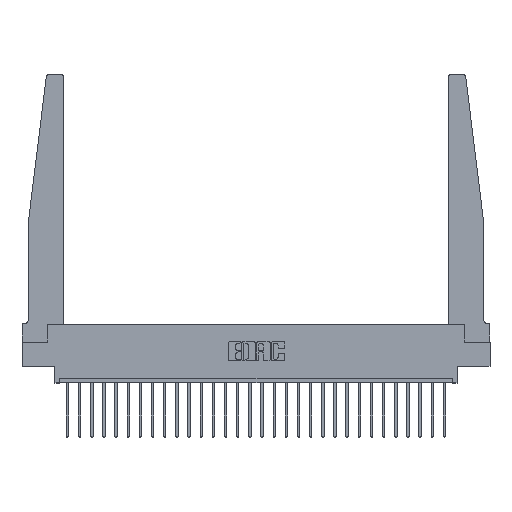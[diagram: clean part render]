
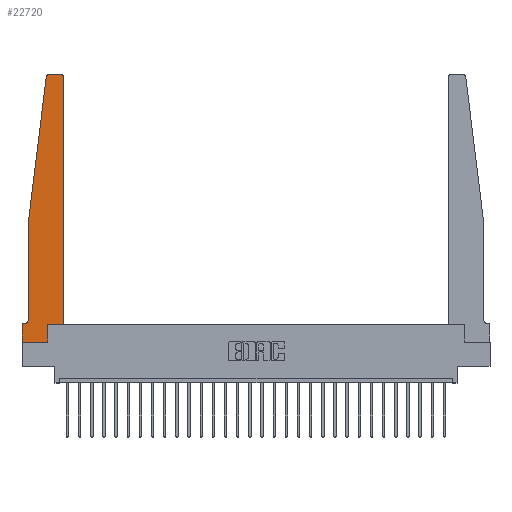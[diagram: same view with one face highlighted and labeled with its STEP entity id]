
A CAD part, top view. The second image highlights one B-rep face of the part: STEP entity #22720.
In plain terms, the highlighted planar face has unit normal (0, 0, 1).
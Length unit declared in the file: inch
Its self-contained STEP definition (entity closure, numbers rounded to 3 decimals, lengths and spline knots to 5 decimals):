
#14 = AXIS2_PLACEMENT_3D ( 'NONE', #17713, #17983, #10589 ) ;
#166 = VERTEX_POINT ( 'NONE', #11202 ) ;
#487 = CARTESIAN_POINT ( 'NONE',  ( 0., 0.1875, 0.37 ) ) ;
#514 = VECTOR ( 'NONE', #20784, 39.37008 ) ;
#967 = VERTEX_POINT ( 'NONE', #8251 ) ;
#980 = ORIENTED_EDGE ( 'NONE', *, *, #1499, .T. ) ;
#1088 = LINE ( 'NONE', #23328, #3349 ) ;
#1499 = EDGE_CURVE ( 'NONE', #7745, #23805, #2889, .T. ) ;
#1550 = CARTESIAN_POINT ( 'NONE',  ( 0.25, 2.75, 0.37 ) ) ;
#1718 = AXIS2_PLACEMENT_3D ( 'NONE', #17797, #5734, #7734 ) ;
#1738 = LINE ( 'NONE', #13025, #6844 ) ;
#2017 = ORIENTED_EDGE ( 'NONE', *, *, #8646, .T. ) ;
#2110 = DIRECTION ( 'NONE',  ( -1., 0., 0. ) ) ;
#2233 = VECTOR ( 'NONE', #14215, 39.37008 ) ;
#2363 = ORIENTED_EDGE ( 'NONE', *, *, #16042, .T. ) ;
#2469 = DIRECTION ( 'NONE',  ( 0., 0., 1. ) ) ;
#2528 = CARTESIAN_POINT ( 'NONE',  ( 0., 0., 0.37 ) ) ;
#2587 = VECTOR ( 'NONE', #2110, 39.37008 ) ;
#2889 = LINE ( 'NONE', #1550, #2587 ) ;
#3087 = ORIENTED_EDGE ( 'NONE', *, *, #20840, .T. ) ;
#3349 = VECTOR ( 'NONE', #17210, 39.37008 ) ;
#4024 = LINE ( 'NONE', #2528, #514 ) ;
#4312 = VECTOR ( 'NONE', #16308, 39.37008 ) ;
#4846 = EDGE_CURVE ( 'NONE', #10331, #13858, #1738, .T. ) ;
#5045 = EDGE_CURVE ( 'NONE', #23805, #17679, #9657, .T. ) ;
#5103 = ORIENTED_EDGE ( 'NONE', *, *, #4846, .T. ) ;
#5146 = DIRECTION ( 'NONE',  ( 0., 1., 0. ) ) ;
#5177 = VECTOR ( 'NONE', #21543, 39.37008 ) ;
#5707 = EDGE_CURVE ( 'NONE', #23766, #21715, #9662, .T. ) ;
#5734 = DIRECTION ( 'NONE',  ( 0., 0., -1. ) ) ;
#5841 = VERTEX_POINT ( 'NONE', #16495 ) ;
#5907 = EDGE_CURVE ( 'NONE', #17679, #967, #1088, .T. ) ;
#6087 = ORIENTED_EDGE ( 'NONE', *, *, #5907, .T. ) ;
#6761 = ORIENTED_EDGE ( 'NONE', *, *, #5707, .T. ) ;
#6844 = VECTOR ( 'NONE', #12948, 39.37008 ) ;
#7000 = EDGE_CURVE ( 'NONE', #967, #19310, #20351, .T. ) ;
#7734 = DIRECTION ( 'NONE',  ( -1., 0., 0. ) ) ;
#7745 = VERTEX_POINT ( 'NONE', #17360 ) ;
#7827 = PLANE ( 'NONE',  #14 ) ;
#7843 = CIRCLE ( 'NONE', #19512, 0.03 ) ;
#8251 = CARTESIAN_POINT ( 'NONE',  ( 0.065, 1.25, 0.37 ) ) ;
#8498 = CARTESIAN_POINT ( 'NONE',  ( 0.425, 0.18, 0.37 ) ) ;
#8646 = EDGE_CURVE ( 'NONE', #166, #23766, #22764, .T. ) ;
#8851 = CARTESIAN_POINT ( 'NONE',  ( 0., 0., 0.37 ) ) ;
#8997 = CARTESIAN_POINT ( 'NONE',  ( 0.27653, 2.75, 0.37 ) ) ;
#9657 = CIRCLE ( 'NONE', #15176, 0.03 ) ;
#9662 = LINE ( 'NONE', #24125, #4312 ) ;
#10255 = DIRECTION ( 'NONE',  ( 0., -1., 0. ) ) ;
#10331 = VERTEX_POINT ( 'NONE', #24391 ) ;
#10589 = DIRECTION ( 'NONE',  ( 1., 0., 0. ) ) ;
#10970 = CARTESIAN_POINT ( 'NONE',  ( 0.065, 1.25, 0.37 ) ) ;
#11202 = CARTESIAN_POINT ( 'NONE',  ( 0.015, 0.1875, 0.37 ) ) ;
#11204 = CARTESIAN_POINT ( 'NONE',  ( 0.2605, 0.18, 0.37 ) ) ;
#11977 = CARTESIAN_POINT ( 'NONE',  ( 0.24675, 2.72367, 0.37 ) ) ;
#12004 = DIRECTION ( 'NONE',  ( 0., 0., 1. ) ) ;
#12233 = EDGE_CURVE ( 'NONE', #13858, #7745, #7843, .T. ) ;
#12539 = CARTESIAN_POINT ( 'NONE',  ( 0.395, 2.72, 0.37 ) ) ;
#12682 = LINE ( 'NONE', #8498, #2233 ) ;
#12948 = DIRECTION ( 'NONE',  ( 0., 1., 0. ) ) ;
#13025 = CARTESIAN_POINT ( 'NONE',  ( 0.425, 0.18, 0.37 ) ) ;
#13488 = CARTESIAN_POINT ( 'NONE',  ( 0.065, 0.1875, 0.37 ) ) ;
#13842 = CIRCLE ( 'NONE', #1718, 0.05 ) ;
#13858 = VERTEX_POINT ( 'NONE', #22881 ) ;
#14085 = ORIENTED_EDGE ( 'NONE', *, *, #24437, .T. ) ;
#14215 = DIRECTION ( 'NONE',  ( 1., 0., 0. ) ) ;
#14817 = DIRECTION ( 'NONE',  ( 1., 0., 0. ) ) ;
#15176 = AXIS2_PLACEMENT_3D ( 'NONE', #23848, #12004, #16210 ) ;
#16042 = EDGE_CURVE ( 'NONE', #21715, #5841, #4024, .T. ) ;
#16210 = DIRECTION ( 'NONE',  ( 1., 0., 0. ) ) ;
#16308 = DIRECTION ( 'NONE',  ( 0., -1., 0. ) ) ;
#16495 = CARTESIAN_POINT ( 'NONE',  ( 0.2605, 0., 0.37 ) ) ;
#16798 = ORIENTED_EDGE ( 'NONE', *, *, #19113, .T. ) ;
#16867 = LINE ( 'NONE', #17123, #19986 ) ;
#17123 = CARTESIAN_POINT ( 'NONE',  ( 0.2605, 0.18, 0.37 ) ) ;
#17210 = DIRECTION ( 'NONE',  ( -0.122, -0.992, 0. ) ) ;
#17360 = CARTESIAN_POINT ( 'NONE',  ( 0.395, 2.75, 0.37 ) ) ;
#17576 = ORIENTED_EDGE ( 'NONE', *, *, #12233, .T. ) ;
#17679 = VERTEX_POINT ( 'NONE', #11977 ) ;
#17713 = CARTESIAN_POINT ( 'NONE',  ( 0., 0.1875, 0.37 ) ) ;
#17797 = CARTESIAN_POINT ( 'NONE',  ( 0.015, 0.2375, 0.37 ) ) ;
#17971 = ORIENTED_EDGE ( 'NONE', *, *, #5045, .T. ) ;
#17983 = DIRECTION ( 'NONE',  ( 0., 0., 1. ) ) ;
#18337 = ORIENTED_EDGE ( 'NONE', *, *, #7000, .T. ) ;
#19113 = EDGE_CURVE ( 'NONE', #25471, #10331, #12682, .T. ) ;
#19310 = VERTEX_POINT ( 'NONE', #25439 ) ;
#19512 = AXIS2_PLACEMENT_3D ( 'NONE', #12539, #2469, #14817 ) ;
#19979 = EDGE_LOOP ( 'NONE', ( #980, #17971, #6087, #18337, #14085, #2017, #6761, #2363, #3087, #16798, #5103, #17576 ) ) ;
#19986 = VECTOR ( 'NONE', #5146, 39.37008 ) ;
#20351 = LINE ( 'NONE', #10970, #22203 ) ;
#20784 = DIRECTION ( 'NONE',  ( 1., 0., 0. ) ) ;
#20840 = EDGE_CURVE ( 'NONE', #5841, #25471, #16867, .T. ) ;
#21543 = DIRECTION ( 'NONE',  ( -1., 0., 0. ) ) ;
#21715 = VERTEX_POINT ( 'NONE', #8851 ) ;
#22203 = VECTOR ( 'NONE', #10255, 39.37008 ) ;
#22720 = ADVANCED_FACE ( 'NONE', ( #25206 ), #7827, .T. ) ;
#22764 = LINE ( 'NONE', #13488, #5177 ) ;
#22881 = CARTESIAN_POINT ( 'NONE',  ( 0.425, 2.72, 0.37 ) ) ;
#23328 = CARTESIAN_POINT ( 'NONE',  ( 0.065, 1.25, 0.37 ) ) ;
#23766 = VERTEX_POINT ( 'NONE', #487 ) ;
#23805 = VERTEX_POINT ( 'NONE', #8997 ) ;
#23848 = CARTESIAN_POINT ( 'NONE',  ( 0.27653, 2.72, 0.37 ) ) ;
#24125 = CARTESIAN_POINT ( 'NONE',  ( 0., 0., 0.37 ) ) ;
#24391 = CARTESIAN_POINT ( 'NONE',  ( 0.425, 0.18, 0.37 ) ) ;
#24437 = EDGE_CURVE ( 'NONE', #19310, #166, #13842, .T. ) ;
#25206 = FACE_OUTER_BOUND ( 'NONE', #19979, .T. ) ;
#25439 = CARTESIAN_POINT ( 'NONE',  ( 0.065, 0.2375, 0.37 ) ) ;
#25471 = VERTEX_POINT ( 'NONE', #11204 ) ;
